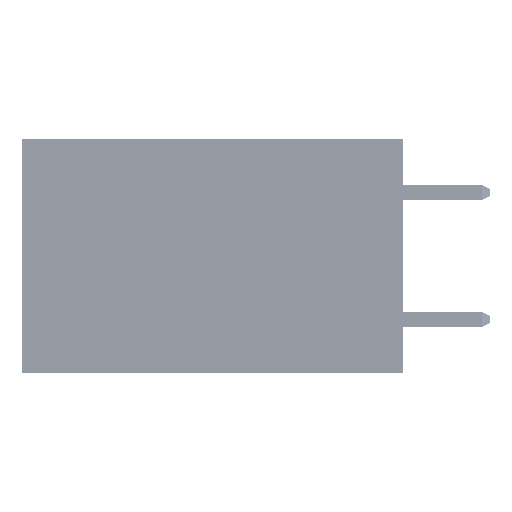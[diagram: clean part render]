
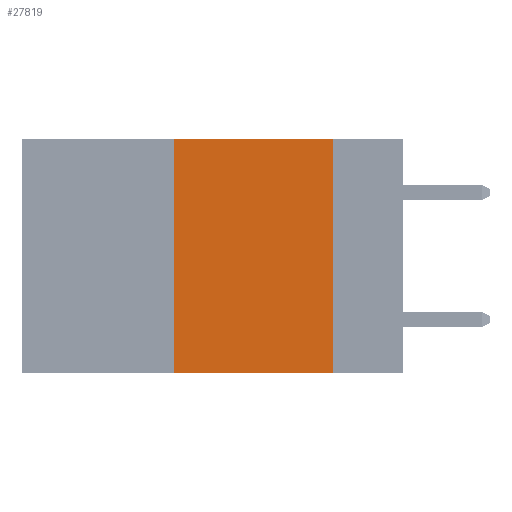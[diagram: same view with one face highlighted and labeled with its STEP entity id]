
A CAD part, left-side view. The second image highlights one B-rep face of the part: STEP entity #27819.
In plain terms, the highlighted planar face has unit normal (-1, 0, 0).
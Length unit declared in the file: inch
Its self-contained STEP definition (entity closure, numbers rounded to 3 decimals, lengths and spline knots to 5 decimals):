
#152 = DIRECTION ( 'NONE',  ( 0., 0., -1. ) ) ;
#1327 = VECTOR ( 'NONE', #3662, 39.37008 ) ;
#1408 = DIRECTION ( 'NONE',  ( 1., 0., 0. ) ) ;
#1827 = VERTEX_POINT ( 'NONE', #22424 ) ;
#1917 = ORIENTED_EDGE ( 'NONE', *, *, #3324, .F. ) ;
#2273 = LINE ( 'NONE', #5741, #21193 ) ;
#2575 = ORIENTED_EDGE ( 'NONE', *, *, #29045, .F. ) ;
#3324 = EDGE_CURVE ( 'NONE', #29071, #18156, #2273, .T. ) ;
#3415 = LINE ( 'NONE', #33380, #1327 ) ;
#3662 = DIRECTION ( 'NONE',  ( 0., -1., 0. ) ) ;
#5741 = CARTESIAN_POINT ( 'NONE',  ( 0., 0.36, 0. ) ) ;
#6071 = VECTOR ( 'NONE', #152, 39.37008 ) ;
#8370 = EDGE_CURVE ( 'NONE', #29071, #29264, #12120, .T. ) ;
#8816 = EDGE_LOOP ( 'NONE', ( #29124, #2575, #1917, #23174 ) ) ;
#9045 = CARTESIAN_POINT ( 'NONE',  ( 0., 0.11, -0.37 ) ) ;
#9290 = FACE_OUTER_BOUND ( 'NONE', #8816, .T. ) ;
#12120 = LINE ( 'NONE', #19492, #43862 ) ;
#16991 = DIRECTION ( 'NONE',  ( 0., 0., 1. ) ) ;
#18156 = VERTEX_POINT ( 'NONE', #37377 ) ;
#19492 = CARTESIAN_POINT ( 'NONE',  ( 0., 0.6, -0.37 ) ) ;
#20297 = PLANE ( 'NONE',  #43298 ) ;
#20776 = CARTESIAN_POINT ( 'NONE',  ( 0., 0.6, 0. ) ) ;
#21193 = VECTOR ( 'NONE', #16991, 39.37008 ) ;
#22424 = CARTESIAN_POINT ( 'NONE',  ( 0., 0.11, 0. ) ) ;
#23174 = ORIENTED_EDGE ( 'NONE', *, *, #8370, .T. ) ;
#24705 = DIRECTION ( 'NONE',  ( 0., 0., -1. ) ) ;
#26491 = CARTESIAN_POINT ( 'NONE',  ( 0., 0.36, -0.37 ) ) ;
#27819 = ADVANCED_FACE ( 'NONE', ( #9290 ), #20297, .F. ) ;
#29045 = EDGE_CURVE ( 'NONE', #18156, #1827, #3415, .T. ) ;
#29071 = VERTEX_POINT ( 'NONE', #26491 ) ;
#29124 = ORIENTED_EDGE ( 'NONE', *, *, #34823, .F. ) ;
#29264 = VERTEX_POINT ( 'NONE', #9045 ) ;
#33380 = CARTESIAN_POINT ( 'NONE',  ( 0., 0.6, 0. ) ) ;
#33986 = DIRECTION ( 'NONE',  ( 0., -1., 0. ) ) ;
#34823 = EDGE_CURVE ( 'NONE', #1827, #29264, #45094, .T. ) ;
#37377 = CARTESIAN_POINT ( 'NONE',  ( 0., 0.36, 0. ) ) ;
#43298 = AXIS2_PLACEMENT_3D ( 'NONE', #20776, #1408, #24705 ) ;
#43862 = VECTOR ( 'NONE', #33986, 39.37008 ) ;
#45094 = LINE ( 'NONE', #48286, #6071 ) ;
#48286 = CARTESIAN_POINT ( 'NONE',  ( 0., 0.11, 0. ) ) ;
